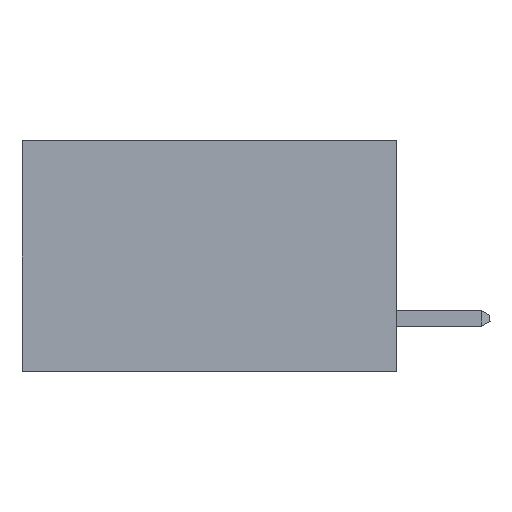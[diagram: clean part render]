
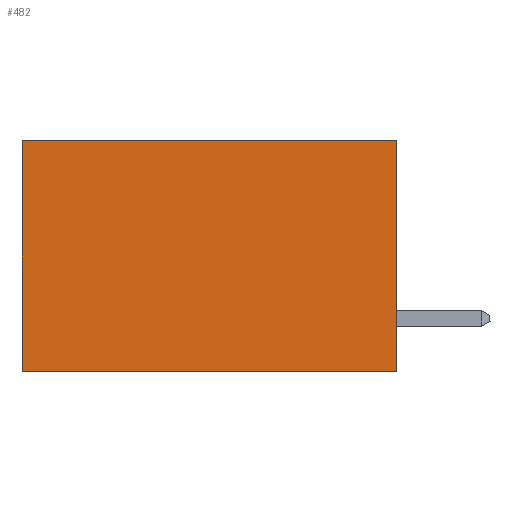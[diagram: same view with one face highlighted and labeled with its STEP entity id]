
A CAD part, left-side view. The second image highlights one B-rep face of the part: STEP entity #482.
In plain terms, the highlighted planar face has unit normal (-1, 0, 0).
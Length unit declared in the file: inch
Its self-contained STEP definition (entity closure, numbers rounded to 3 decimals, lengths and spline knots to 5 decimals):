
#48 = DIRECTION ( 'NONE',  ( 0., 1., 0. ) ) ;
#77 = CARTESIAN_POINT ( 'NONE',  ( 0.2615, 0., -0.37 ) ) ;
#168 = DIRECTION ( 'NONE',  ( 1., 0., 0. ) ) ;
#482 = ADVANCED_FACE ( 'NONE', ( #10945 ), #10650, .F. ) ;
#626 = CARTESIAN_POINT ( 'NONE',  ( 0.2615, 0., -0.37 ) ) ;
#912 = VECTOR ( 'NONE', #4702, 39.37008 ) ;
#1415 = VERTEX_POINT ( 'NONE', #3308 ) ;
#1727 = DIRECTION ( 'NONE',  ( 0., 1., 0. ) ) ;
#2624 = VERTEX_POINT ( 'NONE', #77 ) ;
#2809 = CARTESIAN_POINT ( 'NONE',  ( 0.2615, 0.6, -0.37 ) ) ;
#3308 = CARTESIAN_POINT ( 'NONE',  ( 0.2615, 0., 0. ) ) ;
#3432 = CARTESIAN_POINT ( 'NONE',  ( 0.2615, 0., -0.37 ) ) ;
#4164 = EDGE_CURVE ( 'NONE', #1415, #2624, #11957, .T. ) ;
#4382 = VECTOR ( 'NONE', #48, 39.37008 ) ;
#4702 = DIRECTION ( 'NONE',  ( 0., 0., -1. ) ) ;
#5378 = LINE ( 'NONE', #6460, #4382 ) ;
#5572 = ORIENTED_EDGE ( 'NONE', *, *, #4164, .F. ) ;
#6207 = EDGE_CURVE ( 'NONE', #1415, #9098, #5378, .T. ) ;
#6460 = CARTESIAN_POINT ( 'NONE',  ( 0.2615, 0., 0. ) ) ;
#6476 = EDGE_LOOP ( 'NONE', ( #13814, #10875, #5572, #12311 ) ) ;
#6540 = EDGE_CURVE ( 'NONE', #9098, #13143, #12321, .T. ) ;
#6568 = DIRECTION ( 'NONE',  ( 0., 0., -1. ) ) ;
#6669 = CARTESIAN_POINT ( 'NONE',  ( 0.2615, 0.6, -0.37 ) ) ;
#6871 = CARTESIAN_POINT ( 'NONE',  ( 0.2615, 0., -0.37 ) ) ;
#7696 = AXIS2_PLACEMENT_3D ( 'NONE', #3432, #168, #9819 ) ;
#8701 = CARTESIAN_POINT ( 'NONE',  ( 0.2615, 0.6, 0. ) ) ;
#9098 = VERTEX_POINT ( 'NONE', #8701 ) ;
#9184 = LINE ( 'NONE', #626, #9677 ) ;
#9677 = VECTOR ( 'NONE', #1727, 39.37008 ) ;
#9819 = DIRECTION ( 'NONE',  ( 0., 0., -1. ) ) ;
#10650 = PLANE ( 'NONE',  #7696 ) ;
#10875 = ORIENTED_EDGE ( 'NONE', *, *, #13537, .F. ) ;
#10945 = FACE_OUTER_BOUND ( 'NONE', #6476, .T. ) ;
#11452 = VECTOR ( 'NONE', #6568, 39.37008 ) ;
#11957 = LINE ( 'NONE', #6871, #11452 ) ;
#12311 = ORIENTED_EDGE ( 'NONE', *, *, #6207, .T. ) ;
#12321 = LINE ( 'NONE', #6669, #912 ) ;
#13143 = VERTEX_POINT ( 'NONE', #2809 ) ;
#13537 = EDGE_CURVE ( 'NONE', #2624, #13143, #9184, .T. ) ;
#13814 = ORIENTED_EDGE ( 'NONE', *, *, #6540, .T. ) ;
